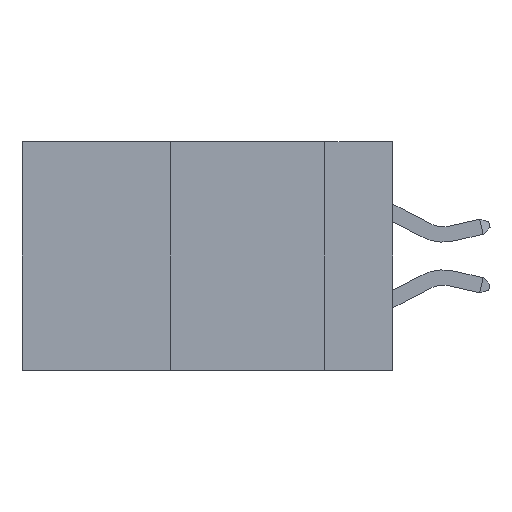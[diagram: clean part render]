
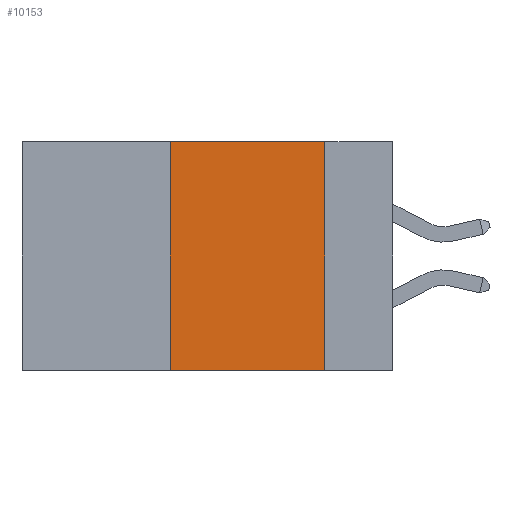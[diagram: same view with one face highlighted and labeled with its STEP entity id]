
A CAD part, left-side view. The second image highlights one B-rep face of the part: STEP entity #10153.
In plain terms, the highlighted planar face has unit normal (-1, 0, 0).
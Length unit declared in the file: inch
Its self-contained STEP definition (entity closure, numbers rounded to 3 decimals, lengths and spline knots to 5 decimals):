
#702 = DIRECTION ( 'NONE',  ( 1., 0., 0. ) ) ;
#2954 = CARTESIAN_POINT ( 'NONE',  ( 0., 0.36, -0.37 ) ) ;
#3761 = LINE ( 'NONE', #7322, #10037 ) ;
#5378 = AXIS2_PLACEMENT_3D ( 'NONE', #39192, #702, #16904 ) ;
#6706 = DIRECTION ( 'NONE',  ( 0., -1., 0. ) ) ;
#7322 = CARTESIAN_POINT ( 'NONE',  ( 0., 0.11, 0. ) ) ;
#8819 = VERTEX_POINT ( 'NONE', #2954 ) ;
#9788 = VECTOR ( 'NONE', #32328, 39.37008 ) ;
#9870 = LINE ( 'NONE', #32170, #24688 ) ;
#10025 = CARTESIAN_POINT ( 'NONE',  ( 0., 0.6, 0. ) ) ;
#10037 = VECTOR ( 'NONE', #30060, 39.37008 ) ;
#10153 = ADVANCED_FACE ( 'NONE', ( #16691 ), #29530, .F. ) ;
#13372 = EDGE_CURVE ( 'NONE', #8819, #22143, #27571, .T. ) ;
#15151 = DIRECTION ( 'NONE',  ( 0., 0., 1. ) ) ;
#16641 = ORIENTED_EDGE ( 'NONE', *, *, #19768, .F. ) ;
#16691 = FACE_OUTER_BOUND ( 'NONE', #24829, .T. ) ;
#16904 = DIRECTION ( 'NONE',  ( 0., 0., -1. ) ) ;
#17678 = EDGE_CURVE ( 'NONE', #8819, #19929, #9870, .T. ) ;
#19768 = EDGE_CURVE ( 'NONE', #30258, #19929, #3761, .T. ) ;
#19929 = VERTEX_POINT ( 'NONE', #39723 ) ;
#21211 = ORIENTED_EDGE ( 'NONE', *, *, #29654, .F. ) ;
#22143 = VERTEX_POINT ( 'NONE', #35661 ) ;
#22387 = ORIENTED_EDGE ( 'NONE', *, *, #17678, .T. ) ;
#24688 = VECTOR ( 'NONE', #6706, 39.37008 ) ;
#24829 = EDGE_LOOP ( 'NONE', ( #16641, #21211, #37278, #22387 ) ) ;
#27571 = LINE ( 'NONE', #37038, #40002 ) ;
#29530 = PLANE ( 'NONE',  #5378 ) ;
#29654 = EDGE_CURVE ( 'NONE', #22143, #30258, #36076, .T. ) ;
#30060 = DIRECTION ( 'NONE',  ( 0., 0., -1. ) ) ;
#30258 = VERTEX_POINT ( 'NONE', #37227 ) ;
#32170 = CARTESIAN_POINT ( 'NONE',  ( 0., 0.6, -0.37 ) ) ;
#32328 = DIRECTION ( 'NONE',  ( 0., -1., 0. ) ) ;
#35661 = CARTESIAN_POINT ( 'NONE',  ( 0., 0.36, 0. ) ) ;
#36076 = LINE ( 'NONE', #10025, #9788 ) ;
#37038 = CARTESIAN_POINT ( 'NONE',  ( 0., 0.36, 0. ) ) ;
#37227 = CARTESIAN_POINT ( 'NONE',  ( 0., 0.11, 0. ) ) ;
#37278 = ORIENTED_EDGE ( 'NONE', *, *, #13372, .F. ) ;
#39192 = CARTESIAN_POINT ( 'NONE',  ( 0., 0.6, 0. ) ) ;
#39723 = CARTESIAN_POINT ( 'NONE',  ( 0., 0.11, -0.37 ) ) ;
#40002 = VECTOR ( 'NONE', #15151, 39.37008 ) ;
